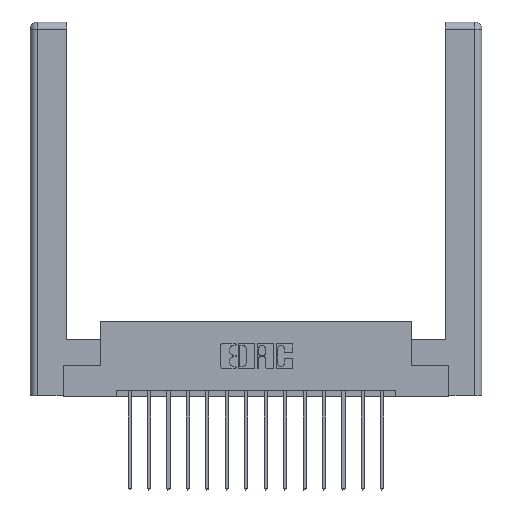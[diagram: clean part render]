
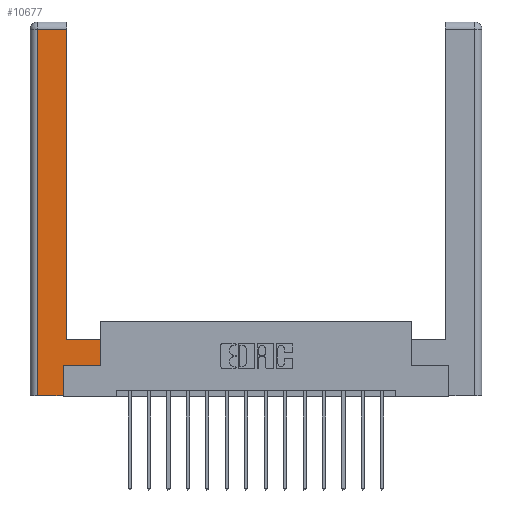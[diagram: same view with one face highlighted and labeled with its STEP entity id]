
A CAD part, top view. The second image highlights one B-rep face of the part: STEP entity #10677.
In plain terms, the highlighted planar face has unit normal (0, 0, 1).
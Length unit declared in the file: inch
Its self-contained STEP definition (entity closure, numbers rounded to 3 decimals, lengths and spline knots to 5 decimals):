
#76 = DIRECTION ( 'NONE',  ( -1., 0., 0. ) ) ;
#85 = ORIENTED_EDGE ( 'NONE', *, *, #11690, .T. ) ;
#117 = EDGE_CURVE ( 'NONE', #9345, #6121, #14199, .T. ) ;
#118 = DIRECTION ( 'NONE',  ( -1., 0., 0. ) ) ;
#700 = ORIENTED_EDGE ( 'NONE', *, *, #13377, .T. ) ;
#779 = VERTEX_POINT ( 'NONE', #11888 ) ;
#2352 = LINE ( 'NONE', #2859, #10831 ) ;
#2479 = LINE ( 'NONE', #13604, #15955 ) ;
#2524 = VECTOR ( 'NONE', #10104, 39.37008 ) ;
#2859 = CARTESIAN_POINT ( 'NONE',  ( 0.565, 0.45, 0. ) ) ;
#3002 = LINE ( 'NONE', #8112, #10464 ) ;
#3046 = CARTESIAN_POINT ( 'NONE',  ( 0.265, 0., 0. ) ) ;
#3076 = ORIENTED_EDGE ( 'NONE', *, *, #8808, .T. ) ;
#3124 = DIRECTION ( 'NONE',  ( 0., 1., 0. ) ) ;
#3174 = VERTEX_POINT ( 'NONE', #11493 ) ;
#3429 = VECTOR ( 'NONE', #15263, 39.37008 ) ;
#3544 = CARTESIAN_POINT ( 'NONE',  ( 0.565, 0.245, 0. ) ) ;
#4224 = EDGE_CURVE ( 'NONE', #4783, #6057, #16367, .T. ) ;
#4245 = EDGE_CURVE ( 'NONE', #6057, #9345, #2479, .T. ) ;
#4306 = CARTESIAN_POINT ( 'NONE',  ( 0.565, 0.245, 0. ) ) ;
#4764 = ORIENTED_EDGE ( 'NONE', *, *, #12271, .T. ) ;
#4783 = VERTEX_POINT ( 'NONE', #7680 ) ;
#6004 = VECTOR ( 'NONE', #13838, 39.37008 ) ;
#6057 = VERTEX_POINT ( 'NONE', #3046 ) ;
#6121 = VERTEX_POINT ( 'NONE', #3544 ) ;
#6286 = CARTESIAN_POINT ( 'NONE',  ( 0.0615, 0., 0. ) ) ;
#6444 = EDGE_CURVE ( 'NONE', #779, #3174, #3002, .T. ) ;
#6726 = VECTOR ( 'NONE', #8780, 39.37008 ) ;
#6747 = PLANE ( 'NONE',  #10993 ) ;
#7544 = LINE ( 'NONE', #8674, #6726 ) ;
#7680 = CARTESIAN_POINT ( 'NONE',  ( 0.0615, 0., 0. ) ) ;
#7911 = ORIENTED_EDGE ( 'NONE', *, *, #4245, .T. ) ;
#8112 = CARTESIAN_POINT ( 'NONE',  ( 0.295, 0.45, 0. ) ) ;
#8408 = CARTESIAN_POINT ( 'NONE',  ( 0.265, 0., 0. ) ) ;
#8674 = CARTESIAN_POINT ( 'NONE',  ( 0.295, 3., 0. ) ) ;
#8780 = DIRECTION ( 'NONE',  ( 0., 1., 0. ) ) ;
#8783 = CARTESIAN_POINT ( 'NONE',  ( 0.265, 0.245, 0. ) ) ;
#8808 = EDGE_CURVE ( 'NONE', #6121, #779, #2352, .T. ) ;
#9345 = VERTEX_POINT ( 'NONE', #8783 ) ;
#10104 = DIRECTION ( 'NONE',  ( 0., -1., 0. ) ) ;
#10464 = VECTOR ( 'NONE', #13892, 39.37008 ) ;
#10629 = DIRECTION ( 'NONE',  ( 0., 1., 0. ) ) ;
#10657 = DIRECTION ( 'NONE',  ( 0., 0., -1. ) ) ;
#10677 = ADVANCED_FACE ( 'NONE', ( #14067 ), #6747, .F. ) ;
#10804 = VERTEX_POINT ( 'NONE', #14423 ) ;
#10831 = VECTOR ( 'NONE', #10629, 39.37008 ) ;
#10993 = AXIS2_PLACEMENT_3D ( 'NONE', #15993, #10657, #118 ) ;
#11019 = VECTOR ( 'NONE', #76, 39.37008 ) ;
#11493 = CARTESIAN_POINT ( 'NONE',  ( 0.295, 0.45, 0. ) ) ;
#11690 = EDGE_CURVE ( 'NONE', #10804, #4783, #14342, .T. ) ;
#11888 = CARTESIAN_POINT ( 'NONE',  ( 0.565, 0.45, 0. ) ) ;
#12054 = LINE ( 'NONE', #14846, #11019 ) ;
#12271 = EDGE_CURVE ( 'NONE', #3174, #14823, #7544, .T. ) ;
#12650 = ORIENTED_EDGE ( 'NONE', *, *, #117, .T. ) ;
#12752 = CARTESIAN_POINT ( 'NONE',  ( 0.295, 2.94, 0. ) ) ;
#13377 = EDGE_CURVE ( 'NONE', #14823, #10804, #12054, .T. ) ;
#13604 = CARTESIAN_POINT ( 'NONE',  ( 0.265, 0.245, 0. ) ) ;
#13838 = DIRECTION ( 'NONE',  ( 1., 0., 0. ) ) ;
#13892 = DIRECTION ( 'NONE',  ( -1., 0., 0. ) ) ;
#14067 = FACE_OUTER_BOUND ( 'NONE', #16992, .T. ) ;
#14199 = LINE ( 'NONE', #4306, #3429 ) ;
#14342 = LINE ( 'NONE', #6286, #2524 ) ;
#14423 = CARTESIAN_POINT ( 'NONE',  ( 0.0615, 2.94, 0. ) ) ;
#14823 = VERTEX_POINT ( 'NONE', #12752 ) ;
#14846 = CARTESIAN_POINT ( 'NONE',  ( 0.0615, 2.94, 0. ) ) ;
#15263 = DIRECTION ( 'NONE',  ( 1., 0., 0. ) ) ;
#15842 = ORIENTED_EDGE ( 'NONE', *, *, #4224, .T. ) ;
#15955 = VECTOR ( 'NONE', #3124, 39.37008 ) ;
#15993 = CARTESIAN_POINT ( 'NONE',  ( 0., 0., 0. ) ) ;
#16367 = LINE ( 'NONE', #8408, #6004 ) ;
#16534 = ORIENTED_EDGE ( 'NONE', *, *, #6444, .T. ) ;
#16992 = EDGE_LOOP ( 'NONE', ( #4764, #700, #85, #15842, #7911, #12650, #3076, #16534 ) ) ;
